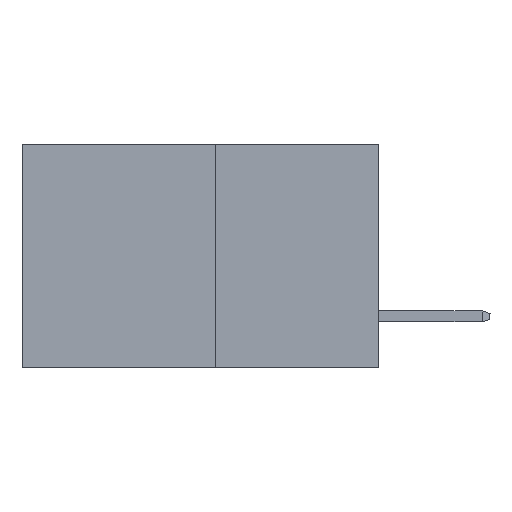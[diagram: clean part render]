
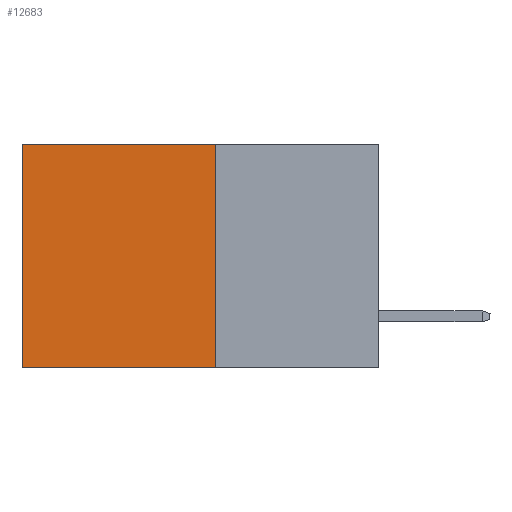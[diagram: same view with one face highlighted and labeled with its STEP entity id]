
A CAD part, left-side view. The second image highlights one B-rep face of the part: STEP entity #12683.
In plain terms, the highlighted planar face has unit normal (-1, 0, 0).
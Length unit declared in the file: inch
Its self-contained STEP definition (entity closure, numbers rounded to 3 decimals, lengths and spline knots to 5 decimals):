
#227 = LINE ( 'NONE', #2685, #5371 ) ;
#550 = CARTESIAN_POINT ( 'NONE',  ( 0.277, 0.27, 0. ) ) ;
#1557 = VECTOR ( 'NONE', #10536, 39.37008 ) ;
#1960 = DIRECTION ( 'NONE',  ( 0., 0., -1. ) ) ;
#2247 = EDGE_CURVE ( 'NONE', #6641, #11423, #5567, .T. ) ;
#2669 = ORIENTED_EDGE ( 'NONE', *, *, #5379, .F. ) ;
#2685 = CARTESIAN_POINT ( 'NONE',  ( 0.277, 0.59, -0.37 ) ) ;
#2995 = ORIENTED_EDGE ( 'NONE', *, *, #8597, .F. ) ;
#3063 = DIRECTION ( 'NONE',  ( 0., 1., 0. ) ) ;
#3532 = CARTESIAN_POINT ( 'NONE',  ( 0.277, 0.27, -0.37 ) ) ;
#3763 = VECTOR ( 'NONE', #3783, 39.37008 ) ;
#3783 = DIRECTION ( 'NONE',  ( 0., 1., 0. ) ) ;
#3993 = CARTESIAN_POINT ( 'NONE',  ( 0.277, 0.27, -0.37 ) ) ;
#4064 = CARTESIAN_POINT ( 'NONE',  ( 0.277, 0.59, 0. ) ) ;
#4202 = FACE_OUTER_BOUND ( 'NONE', #9110, .T. ) ;
#4561 = AXIS2_PLACEMENT_3D ( 'NONE', #3993, #8056, #1960 ) ;
#4959 = CARTESIAN_POINT ( 'NONE',  ( 0.277, 0.27, -0.37 ) ) ;
#5371 = VECTOR ( 'NONE', #7721, 39.37008 ) ;
#5379 = EDGE_CURVE ( 'NONE', #7594, #6102, #11762, .T. ) ;
#5567 = LINE ( 'NONE', #7834, #8294 ) ;
#6102 = VERTEX_POINT ( 'NONE', #12918 ) ;
#6641 = VERTEX_POINT ( 'NONE', #550 ) ;
#6643 = LINE ( 'NONE', #3532, #1557 ) ;
#7594 = VERTEX_POINT ( 'NONE', #4959 ) ;
#7721 = DIRECTION ( 'NONE',  ( 0., 0., -1. ) ) ;
#7834 = CARTESIAN_POINT ( 'NONE',  ( 0.277, 0.27, 0. ) ) ;
#8056 = DIRECTION ( 'NONE',  ( 1., 0., 0. ) ) ;
#8294 = VECTOR ( 'NONE', #3063, 39.37008 ) ;
#8597 = EDGE_CURVE ( 'NONE', #6641, #7594, #6643, .T. ) ;
#8687 = EDGE_CURVE ( 'NONE', #11423, #6102, #227, .T. ) ;
#9110 = EDGE_LOOP ( 'NONE', ( #10354, #2669, #2995, #10966 ) ) ;
#9792 = CARTESIAN_POINT ( 'NONE',  ( 0.277, 0.27, -0.37 ) ) ;
#10354 = ORIENTED_EDGE ( 'NONE', *, *, #8687, .T. ) ;
#10536 = DIRECTION ( 'NONE',  ( 0., 0., -1. ) ) ;
#10966 = ORIENTED_EDGE ( 'NONE', *, *, #2247, .T. ) ;
#10969 = PLANE ( 'NONE',  #4561 ) ;
#11423 = VERTEX_POINT ( 'NONE', #4064 ) ;
#11762 = LINE ( 'NONE', #9792, #3763 ) ;
#12683 = ADVANCED_FACE ( 'NONE', ( #4202 ), #10969, .F. ) ;
#12918 = CARTESIAN_POINT ( 'NONE',  ( 0.277, 0.59, -0.37 ) ) ;
